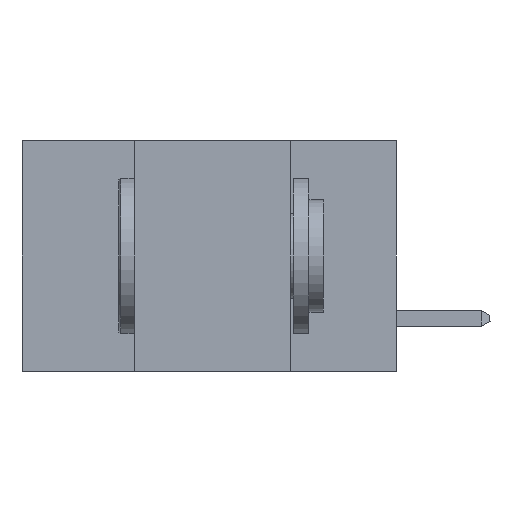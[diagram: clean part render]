
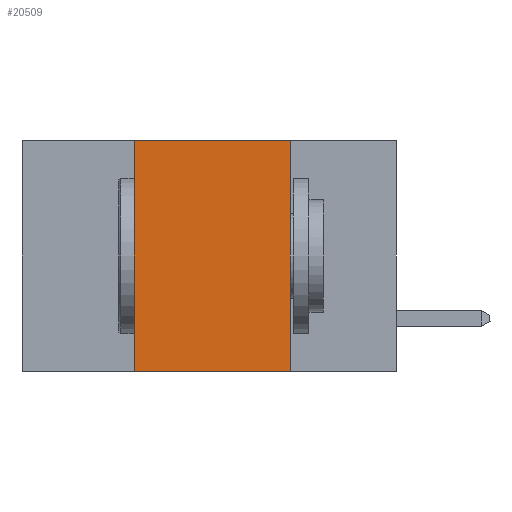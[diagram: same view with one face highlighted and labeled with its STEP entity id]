
A CAD part, left-side view. The second image highlights one B-rep face of the part: STEP entity #20509.
In plain terms, the highlighted planar face has unit normal (-1, 0, 0).
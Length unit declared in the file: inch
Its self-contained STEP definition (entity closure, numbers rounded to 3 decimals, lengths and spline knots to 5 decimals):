
#1705 = CARTESIAN_POINT ( 'NONE',  ( 0., 0.6, 0. ) ) ;
#2169 = CARTESIAN_POINT ( 'NONE',  ( 0., 0.17, 0. ) ) ;
#2635 = LINE ( 'NONE', #6384, #12031 ) ;
#3107 = VERTEX_POINT ( 'NONE', #12249 ) ;
#3231 = CARTESIAN_POINT ( 'NONE',  ( 0., 0.42, 0. ) ) ;
#3739 = LINE ( 'NONE', #3231, #22321 ) ;
#4016 = FACE_OUTER_BOUND ( 'NONE', #12271, .T. ) ;
#4213 = VECTOR ( 'NONE', #12729, 39.37008 ) ;
#4585 = ORIENTED_EDGE ( 'NONE', *, *, #15598, .F. ) ;
#5438 = VERTEX_POINT ( 'NONE', #17709 ) ;
#5589 = PLANE ( 'NONE',  #11237 ) ;
#5620 = EDGE_CURVE ( 'NONE', #8366, #20202, #23262, .T. ) ;
#6342 = EDGE_CURVE ( 'NONE', #5438, #3107, #2635, .T. ) ;
#6384 = CARTESIAN_POINT ( 'NONE',  ( 0., 0.6, 0. ) ) ;
#7474 = DIRECTION ( 'NONE',  ( 0., 0., -1. ) ) ;
#7951 = LINE ( 'NONE', #2169, #17495 ) ;
#8366 = VERTEX_POINT ( 'NONE', #14071 ) ;
#8567 = DIRECTION ( 'NONE',  ( 0., -1., 0. ) ) ;
#10209 = ORIENTED_EDGE ( 'NONE', *, *, #5620, .T. ) ;
#11237 = AXIS2_PLACEMENT_3D ( 'NONE', #1705, #18253, #7474 ) ;
#12031 = VECTOR ( 'NONE', #8567, 39.37008 ) ;
#12249 = CARTESIAN_POINT ( 'NONE',  ( 0., 0.17, 0. ) ) ;
#12271 = EDGE_LOOP ( 'NONE', ( #4585, #22574, #22284, #10209 ) ) ;
#12729 = DIRECTION ( 'NONE',  ( 0., -1., 0. ) ) ;
#12876 = CARTESIAN_POINT ( 'NONE',  ( 0., 0.6, -0.37 ) ) ;
#14071 = CARTESIAN_POINT ( 'NONE',  ( 0., 0.42, -0.37 ) ) ;
#15366 = CARTESIAN_POINT ( 'NONE',  ( 0., 0.17, -0.37 ) ) ;
#15598 = EDGE_CURVE ( 'NONE', #3107, #20202, #7951, .T. ) ;
#16600 = EDGE_CURVE ( 'NONE', #8366, #5438, #3739, .T. ) ;
#16929 = DIRECTION ( 'NONE',  ( 0., 0., -1. ) ) ;
#17495 = VECTOR ( 'NONE', #16929, 39.37008 ) ;
#17709 = CARTESIAN_POINT ( 'NONE',  ( 0., 0.42, 0. ) ) ;
#17875 = DIRECTION ( 'NONE',  ( 0., 0., 1. ) ) ;
#18253 = DIRECTION ( 'NONE',  ( 1., 0., 0. ) ) ;
#20202 = VERTEX_POINT ( 'NONE', #15366 ) ;
#20509 = ADVANCED_FACE ( 'NONE', ( #4016 ), #5589, .F. ) ;
#22284 = ORIENTED_EDGE ( 'NONE', *, *, #16600, .F. ) ;
#22321 = VECTOR ( 'NONE', #17875, 39.37008 ) ;
#22574 = ORIENTED_EDGE ( 'NONE', *, *, #6342, .F. ) ;
#23262 = LINE ( 'NONE', #12876, #4213 ) ;
